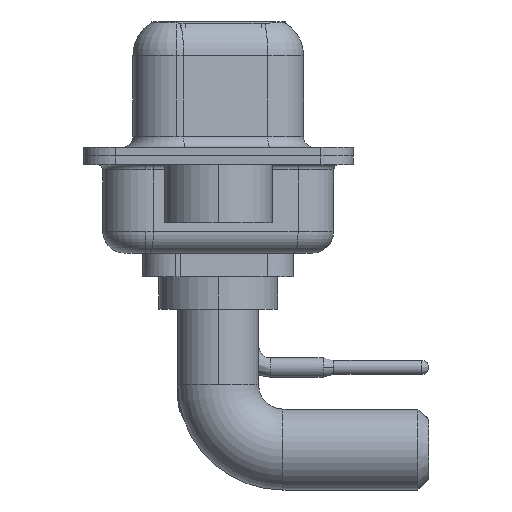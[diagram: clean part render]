
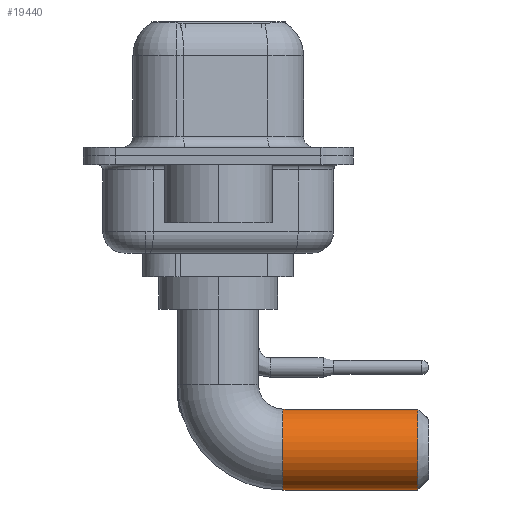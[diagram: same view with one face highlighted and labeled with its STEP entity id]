
A CAD part, left-side view. The second image highlights one B-rep face of the part: STEP entity #19440.
In plain terms, the highlighted cylindrical face has radius 1.875 mm (diameter 3.75 mm), a partial arc.
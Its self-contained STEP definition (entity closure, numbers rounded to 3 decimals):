
#79 = DIRECTION ( 'NONE',  ( 0., 0., -1. ) ) ;
#125 = EDGE_CURVE ( 'NONE', #19616, #1846, #17951, .T. ) ;
#454 = CARTESIAN_POINT ( 'NONE',  ( 0., -3., -4.625 ) ) ;
#514 = AXIS2_PLACEMENT_3D ( 'NONE', #6118, #7867, #79 ) ;
#794 = DIRECTION ( 'NONE',  ( -1., 0., 0. ) ) ;
#1232 = EDGE_CURVE ( 'NONE', #19616, #6602, #7558, .T. ) ;
#1846 = VERTEX_POINT ( 'NONE', #3368 ) ;
#3368 = CARTESIAN_POINT ( 'NONE',  ( 0., -9.25, -4.625 ) ) ;
#3629 = EDGE_CURVE ( 'NONE', #6602, #10956, #23209, .T. ) ;
#4437 = CARTESIAN_POINT ( 'NONE',  ( 0., -9.25, -8.375 ) ) ;
#5520 = CIRCLE ( 'NONE', #9562, 1.875 ) ;
#5619 = EDGE_LOOP ( 'NONE', ( #23574, #17799, #20548, #12418 ) ) ;
#5723 = CYLINDRICAL_SURFACE ( 'NONE', #514, 1.875 ) ;
#6118 = CARTESIAN_POINT ( 'NONE',  ( 0., -3., -6.5 ) ) ;
#6602 = VERTEX_POINT ( 'NONE', #11963 ) ;
#6700 = DIRECTION ( 'NONE',  ( 0., -1., 0. ) ) ;
#7558 = CIRCLE ( 'NONE', #24835, 1.875 ) ;
#7867 = DIRECTION ( 'NONE',  ( 0., -1., 0. ) ) ;
#8524 = DIRECTION ( 'NONE',  ( 0., -1., 0. ) ) ;
#9377 = CARTESIAN_POINT ( 'NONE',  ( 0., -3., -8.375 ) ) ;
#9562 = AXIS2_PLACEMENT_3D ( 'NONE', #15373, #15633, #13361 ) ;
#10956 = VERTEX_POINT ( 'NONE', #4437 ) ;
#11576 = CARTESIAN_POINT ( 'NONE',  ( 0., -3., -4.625 ) ) ;
#11963 = CARTESIAN_POINT ( 'NONE',  ( 0., -3., -8.375 ) ) ;
#12418 = ORIENTED_EDGE ( 'NONE', *, *, #14954, .T. ) ;
#13361 = DIRECTION ( 'NONE',  ( 0., 0., -1. ) ) ;
#14954 = EDGE_CURVE ( 'NONE', #10956, #1846, #5520, .T. ) ;
#15373 = CARTESIAN_POINT ( 'NONE',  ( 0., -9.25, -6.5 ) ) ;
#15540 = DIRECTION ( 'NONE',  ( 0., -1., 0. ) ) ;
#15633 = DIRECTION ( 'NONE',  ( 0., 1., 0. ) ) ;
#17799 = ORIENTED_EDGE ( 'NONE', *, *, #1232, .T. ) ;
#17951 = LINE ( 'NONE', #11576, #21146 ) ;
#19440 = ADVANCED_FACE ( 'NONE', ( #21200 ), #5723, .T. ) ;
#19616 = VERTEX_POINT ( 'NONE', #454 ) ;
#20548 = ORIENTED_EDGE ( 'NONE', *, *, #3629, .T. ) ;
#21146 = VECTOR ( 'NONE', #8524, 1000. ) ;
#21200 = FACE_OUTER_BOUND ( 'NONE', #5619, .T. ) ;
#21664 = CARTESIAN_POINT ( 'NONE',  ( 0., -3., -6.5 ) ) ;
#23209 = LINE ( 'NONE', #9377, #23276 ) ;
#23276 = VECTOR ( 'NONE', #15540, 1000. ) ;
#23574 = ORIENTED_EDGE ( 'NONE', *, *, #125, .F. ) ;
#24835 = AXIS2_PLACEMENT_3D ( 'NONE', #21664, #6700, #794 ) ;
